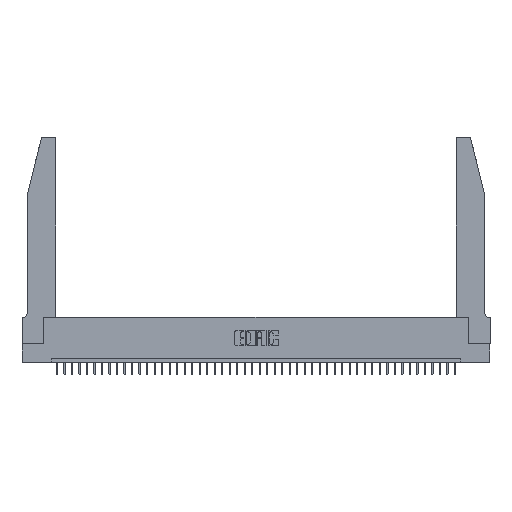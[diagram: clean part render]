
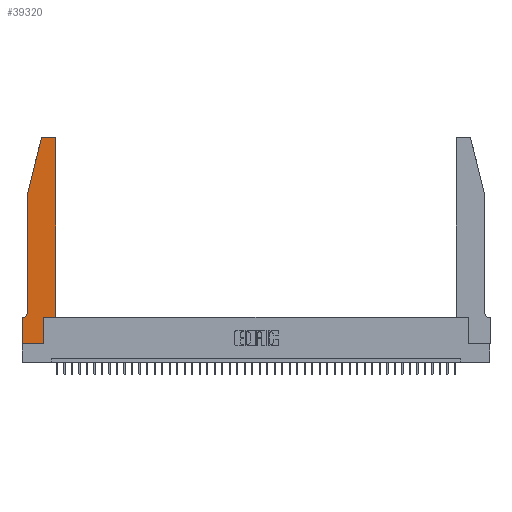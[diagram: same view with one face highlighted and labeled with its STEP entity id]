
A CAD part, top view. The second image highlights one B-rep face of the part: STEP entity #39320.
In plain terms, the highlighted planar face has unit normal (0, 0, 1).
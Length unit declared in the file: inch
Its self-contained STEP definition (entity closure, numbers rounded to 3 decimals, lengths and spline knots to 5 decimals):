
#192 = EDGE_CURVE ( 'NONE', #35043, #12745, #18776, .T. ) ;
#647 = CARTESIAN_POINT ( 'NONE',  ( 0.2865, 0.35, 0.37 ) ) ;
#901 = CARTESIAN_POINT ( 'NONE',  ( 0.4205, 2.72, 0.37 ) ) ;
#933 = LINE ( 'NONE', #33199, #38073 ) ;
#1372 = EDGE_CURVE ( 'NONE', #12745, #23239, #38783, .T. ) ;
#1660 = AXIS2_PLACEMENT_3D ( 'NONE', #901, #20801, #28111 ) ;
#1682 = DIRECTION ( 'NONE',  ( 0., 0., 1. ) ) ;
#2263 = CARTESIAN_POINT ( 'NONE',  ( 0.2605, 2.75, 0.37 ) ) ;
#2275 = ORIENTED_EDGE ( 'NONE', *, *, #192, .T. ) ;
#2756 = DIRECTION ( 'NONE',  ( 0., -1., 0. ) ) ;
#4015 = ORIENTED_EDGE ( 'NONE', *, *, #21170, .T. ) ;
#4770 = CARTESIAN_POINT ( 'NONE',  ( 0., 0.35, 0.37 ) ) ;
#5233 = LINE ( 'NONE', #36533, #32888 ) ;
#6196 = CARTESIAN_POINT ( 'NONE',  ( 0.284, 2.72, 0.37 ) ) ;
#6494 = ORIENTED_EDGE ( 'NONE', *, *, #31928, .T. ) ;
#6693 = EDGE_CURVE ( 'NONE', #23239, #29472, #5233, .T. ) ;
#6722 = DIRECTION ( 'NONE',  ( -0.239, -0.971, 0. ) ) ;
#6788 = CARTESIAN_POINT ( 'NONE',  ( 0., 0., 0.37 ) ) ;
#6972 = VECTOR ( 'NONE', #7218, 39.37008 ) ;
#7218 = DIRECTION ( 'NONE',  ( -1., 0., 0. ) ) ;
#7587 = VERTEX_POINT ( 'NONE', #42564 ) ;
#7928 = EDGE_CURVE ( 'NONE', #25516, #23505, #18333, .T. ) ;
#7933 = VECTOR ( 'NONE', #9472, 39.37008 ) ;
#7978 = CIRCLE ( 'NONE', #34255, 0.03 ) ;
#8191 = CARTESIAN_POINT ( 'NONE',  ( 0.4205, 2.75, 0.37 ) ) ;
#9029 = CARTESIAN_POINT ( 'NONE',  ( 0.4505, 0.35, 0.37 ) ) ;
#9337 = ORIENTED_EDGE ( 'NONE', *, *, #12141, .T. ) ;
#9472 = DIRECTION ( 'NONE',  ( -1., 0., 0. ) ) ;
#9604 = DIRECTION ( 'NONE',  ( 1., 0., 0. ) ) ;
#9745 = CARTESIAN_POINT ( 'NONE',  ( 0.284, 2.75, 0.37 ) ) ;
#9858 = VECTOR ( 'NONE', #32523, 39.37008 ) ;
#11029 = ORIENTED_EDGE ( 'NONE', *, *, #24697, .T. ) ;
#11187 = DIRECTION ( 'NONE',  ( -1., 0., 0. ) ) ;
#11335 = DIRECTION ( 'NONE',  ( 0., 0., -1. ) ) ;
#11507 = CARTESIAN_POINT ( 'NONE',  ( 0., 0., 0.37 ) ) ;
#12141 = EDGE_CURVE ( 'NONE', #31096, #30203, #14990, .T. ) ;
#12170 = ORIENTED_EDGE ( 'NONE', *, *, #1372, .T. ) ;
#12745 = VERTEX_POINT ( 'NONE', #28711 ) ;
#13480 = EDGE_CURVE ( 'NONE', #30203, #15893, #34013, .T. ) ;
#13608 = CARTESIAN_POINT ( 'NONE',  ( 0.0755, 0.35, 0.37 ) ) ;
#13748 = CARTESIAN_POINT ( 'NONE',  ( 0.0755, 2., 0.37 ) ) ;
#14127 = VECTOR ( 'NONE', #22499, 39.37008 ) ;
#14990 = CIRCLE ( 'NONE', #1660, 0.03 ) ;
#15074 = CARTESIAN_POINT ( 'NONE',  ( 0.2865, 0.35, 0.37 ) ) ;
#15481 = EDGE_CURVE ( 'NONE', #27436, #7587, #933, .T. ) ;
#15816 = VERTEX_POINT ( 'NONE', #33193 ) ;
#15893 = VERTEX_POINT ( 'NONE', #9745 ) ;
#15976 = ORIENTED_EDGE ( 'NONE', *, *, #13480, .T. ) ;
#16162 = LINE ( 'NONE', #13748, #21136 ) ;
#16731 = CARTESIAN_POINT ( 'NONE',  ( 0.25487, 2.72718, 0.37 ) ) ;
#18173 = VECTOR ( 'NONE', #29579, 39.37008 ) ;
#18333 = LINE ( 'NONE', #9029, #9858 ) ;
#18776 = CIRCLE ( 'NONE', #27307, 0.07 ) ;
#20198 = DIRECTION ( 'NONE',  ( 0., -1., 0. ) ) ;
#20801 = DIRECTION ( 'NONE',  ( 0., 0., 1. ) ) ;
#20871 = CARTESIAN_POINT ( 'NONE',  ( 0.4505, 0.35, 0.37 ) ) ;
#21136 = VECTOR ( 'NONE', #20198, 39.37008 ) ;
#21170 = EDGE_CURVE ( 'NONE', #23505, #31096, #28565, .T. ) ;
#21711 = ORIENTED_EDGE ( 'NONE', *, *, #27442, .T. ) ;
#22499 = DIRECTION ( 'NONE',  ( 0., 1., 0. ) ) ;
#23239 = VERTEX_POINT ( 'NONE', #33328 ) ;
#23505 = VERTEX_POINT ( 'NONE', #20871 ) ;
#24697 = EDGE_CURVE ( 'NONE', #15816, #25516, #28338, .T. ) ;
#25516 = VERTEX_POINT ( 'NONE', #647 ) ;
#25568 = VECTOR ( 'NONE', #38184, 39.37008 ) ;
#25870 = ORIENTED_EDGE ( 'NONE', *, *, #6693, .T. ) ;
#27307 = AXIS2_PLACEMENT_3D ( 'NONE', #31568, #11335, #11187 ) ;
#27436 = VERTEX_POINT ( 'NONE', #16731 ) ;
#27442 = EDGE_CURVE ( 'NONE', #7587, #35043, #16162, .T. ) ;
#28111 = DIRECTION ( 'NONE',  ( 1., 0., 0. ) ) ;
#28338 = LINE ( 'NONE', #15074, #18173 ) ;
#28401 = PLANE ( 'NONE',  #35971 ) ;
#28565 = LINE ( 'NONE', #42745, #14127 ) ;
#28711 = CARTESIAN_POINT ( 'NONE',  ( 0.0055, 0.35, 0.37 ) ) ;
#29472 = VERTEX_POINT ( 'NONE', #11507 ) ;
#29579 = DIRECTION ( 'NONE',  ( 0., 1., 0. ) ) ;
#30203 = VERTEX_POINT ( 'NONE', #8191 ) ;
#30703 = ORIENTED_EDGE ( 'NONE', *, *, #41938, .T. ) ;
#31096 = VERTEX_POINT ( 'NONE', #43223 ) ;
#31568 = CARTESIAN_POINT ( 'NONE',  ( 0.0055, 0.42, 0.37 ) ) ;
#31928 = EDGE_CURVE ( 'NONE', #15893, #27436, #7978, .T. ) ;
#32159 = EDGE_LOOP ( 'NONE', ( #15976, #6494, #33957, #21711, #2275, #12170, #25870, #30703, #11029, #37982, #4015, #9337 ) ) ;
#32523 = DIRECTION ( 'NONE',  ( 1., 0., 0. ) ) ;
#32888 = VECTOR ( 'NONE', #2756, 39.37008 ) ;
#33193 = CARTESIAN_POINT ( 'NONE',  ( 0.2865, 0., 0.37 ) ) ;
#33199 = CARTESIAN_POINT ( 'NONE',  ( 0.0755, 2., 0.37 ) ) ;
#33328 = CARTESIAN_POINT ( 'NONE',  ( 0., 0.35, 0.37 ) ) ;
#33957 = ORIENTED_EDGE ( 'NONE', *, *, #15481, .T. ) ;
#34013 = LINE ( 'NONE', #2263, #7933 ) ;
#34255 = AXIS2_PLACEMENT_3D ( 'NONE', #6196, #36600, #9604 ) ;
#35043 = VERTEX_POINT ( 'NONE', #35552 ) ;
#35552 = CARTESIAN_POINT ( 'NONE',  ( 0.0755, 0.42, 0.37 ) ) ;
#35971 = AXIS2_PLACEMENT_3D ( 'NONE', #4770, #1682, #38683 ) ;
#36533 = CARTESIAN_POINT ( 'NONE',  ( 0., 0., 0.37 ) ) ;
#36600 = DIRECTION ( 'NONE',  ( 0., 0., 1. ) ) ;
#37711 = FACE_OUTER_BOUND ( 'NONE', #32159, .T. ) ;
#37982 = ORIENTED_EDGE ( 'NONE', *, *, #7928, .T. ) ;
#38073 = VECTOR ( 'NONE', #6722, 39.37008 ) ;
#38184 = DIRECTION ( 'NONE',  ( 1., 0., 0. ) ) ;
#38683 = DIRECTION ( 'NONE',  ( 1., 0., 0. ) ) ;
#38783 = LINE ( 'NONE', #13608, #6972 ) ;
#39320 = ADVANCED_FACE ( 'NONE', ( #37711 ), #28401, .T. ) ;
#41938 = EDGE_CURVE ( 'NONE', #29472, #15816, #42511, .T. ) ;
#42511 = LINE ( 'NONE', #6788, #25568 ) ;
#42564 = CARTESIAN_POINT ( 'NONE',  ( 0.0755, 2., 0.37 ) ) ;
#42745 = CARTESIAN_POINT ( 'NONE',  ( 0.4505, 0.35, 0.37 ) ) ;
#43223 = CARTESIAN_POINT ( 'NONE',  ( 0.4505, 2.72, 0.37 ) ) ;
